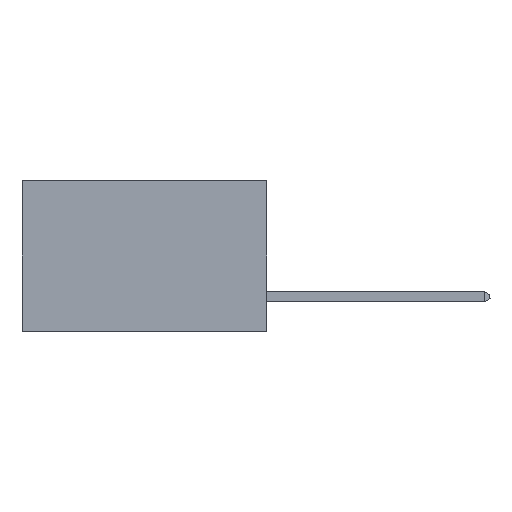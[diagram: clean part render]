
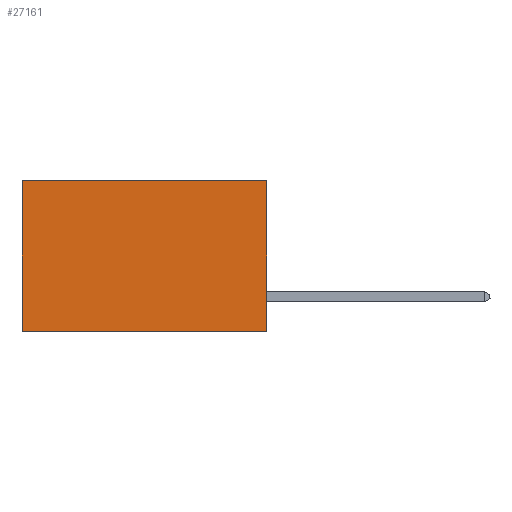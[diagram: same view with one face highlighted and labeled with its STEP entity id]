
A CAD part, left-side view. The second image highlights one B-rep face of the part: STEP entity #27161.
In plain terms, the highlighted planar face has unit normal (-1, 0, 0).
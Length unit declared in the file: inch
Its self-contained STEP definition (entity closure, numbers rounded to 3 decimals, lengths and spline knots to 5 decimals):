
#3112 = VERTEX_POINT ( 'NONE', #34022 ) ;
#4296 = EDGE_CURVE ( 'NONE', #30608, #4611, #32332, .T. ) ;
#4611 = VERTEX_POINT ( 'NONE', #27091 ) ;
#5885 = ORIENTED_EDGE ( 'NONE', *, *, #26456, .T. ) ;
#7699 = DIRECTION ( 'NONE',  ( 0., 0., -1. ) ) ;
#8892 = VECTOR ( 'NONE', #17766, 39.37008 ) ;
#9112 = LINE ( 'NONE', #33636, #27766 ) ;
#9572 = VERTEX_POINT ( 'NONE', #23112 ) ;
#9867 = ORIENTED_EDGE ( 'NONE', *, *, #4296, .F. ) ;
#12546 = EDGE_CURVE ( 'NONE', #4611, #9572, #14552, .T. ) ;
#14197 = EDGE_CURVE ( 'NONE', #30608, #3112, #35463, .T. ) ;
#14283 = DIRECTION ( 'NONE',  ( 1., 0., 0. ) ) ;
#14552 = LINE ( 'NONE', #34309, #8892 ) ;
#14557 = CARTESIAN_POINT ( 'NONE',  ( 0.2875, 0., 0. ) ) ;
#17238 = VECTOR ( 'NONE', #17862, 39.37008 ) ;
#17766 = DIRECTION ( 'NONE',  ( 0., 1., 0. ) ) ;
#17862 = DIRECTION ( 'NONE',  ( 0., 0., -1. ) ) ;
#20440 = FACE_OUTER_BOUND ( 'NONE', #39934, .T. ) ;
#21750 = CARTESIAN_POINT ( 'NONE',  ( 0.2875, 0., 0. ) ) ;
#23112 = CARTESIAN_POINT ( 'NONE',  ( 0.2875, 0.6, -0.37 ) ) ;
#25563 = VECTOR ( 'NONE', #28784, 39.37008 ) ;
#26456 = EDGE_CURVE ( 'NONE', #3112, #9572, #9112, .T. ) ;
#27091 = CARTESIAN_POINT ( 'NONE',  ( 0.2875, 0., -0.37 ) ) ;
#27161 = ADVANCED_FACE ( 'NONE', ( #20440 ), #34305, .F. ) ;
#27761 = CARTESIAN_POINT ( 'NONE',  ( 0.2875, 0., 0. ) ) ;
#27766 = VECTOR ( 'NONE', #7699, 39.37008 ) ;
#28784 = DIRECTION ( 'NONE',  ( 0., 1., 0. ) ) ;
#30608 = VERTEX_POINT ( 'NONE', #42659 ) ;
#32332 = LINE ( 'NONE', #21750, #17238 ) ;
#33636 = CARTESIAN_POINT ( 'NONE',  ( 0.2875, 0.6, 0. ) ) ;
#34022 = CARTESIAN_POINT ( 'NONE',  ( 0.2875, 0.6, 0. ) ) ;
#34082 = AXIS2_PLACEMENT_3D ( 'NONE', #27761, #14283, #37373 ) ;
#34305 = PLANE ( 'NONE',  #34082 ) ;
#34309 = CARTESIAN_POINT ( 'NONE',  ( 0.2875, 0., -0.37 ) ) ;
#35463 = LINE ( 'NONE', #14557, #25563 ) ;
#37373 = DIRECTION ( 'NONE',  ( 0., 0., -1. ) ) ;
#39934 = EDGE_LOOP ( 'NONE', ( #5885, #42520, #9867, #41000 ) ) ;
#41000 = ORIENTED_EDGE ( 'NONE', *, *, #14197, .T. ) ;
#42520 = ORIENTED_EDGE ( 'NONE', *, *, #12546, .F. ) ;
#42659 = CARTESIAN_POINT ( 'NONE',  ( 0.2875, 0., 0. ) ) ;
